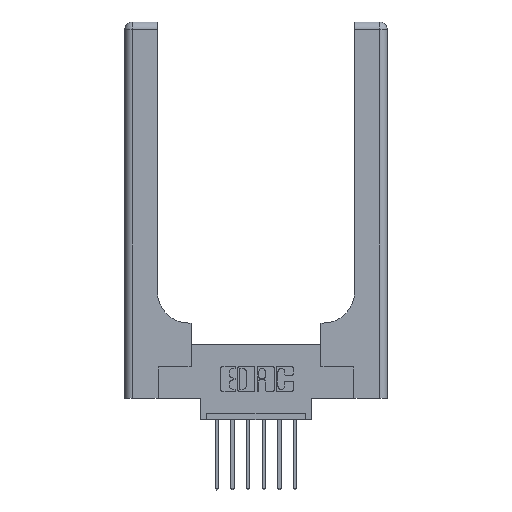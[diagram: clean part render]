
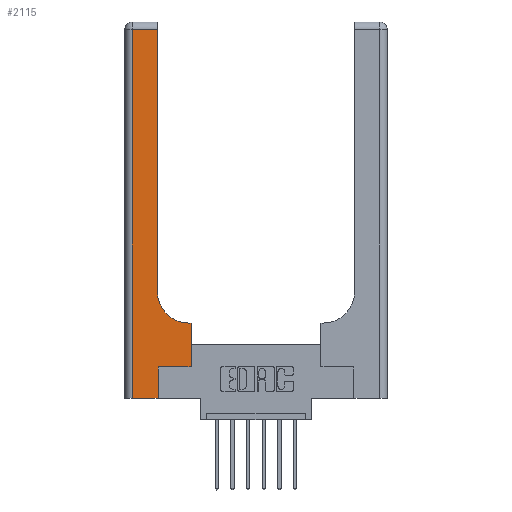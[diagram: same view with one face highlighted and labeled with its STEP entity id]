
A CAD part, top view. The second image highlights one B-rep face of the part: STEP entity #2115.
In plain terms, the highlighted planar face has unit normal (0, 0, 1).
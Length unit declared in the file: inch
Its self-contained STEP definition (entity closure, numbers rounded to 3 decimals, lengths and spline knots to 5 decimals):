
#15 = DIRECTION ( 'NONE',  ( 0., 1., 0. ) ) ;
#78 = CARTESIAN_POINT ( 'NONE',  ( 0., 2.94, 0.37 ) ) ;
#370 = CARTESIAN_POINT ( 'NONE',  ( 0.06, 3., 0.37 ) ) ;
#759 = ORIENTED_EDGE ( 'NONE', *, *, #9715, .T. ) ;
#881 = ORIENTED_EDGE ( 'NONE', *, *, #1555, .T. ) ;
#924 = CARTESIAN_POINT ( 'NONE',  ( 0.528, 0.25, 0.37 ) ) ;
#1103 = LINE ( 'NONE', #5512, #12631 ) ;
#1555 = EDGE_CURVE ( 'NONE', #10380, #11498, #8942, .T. ) ;
#1660 = CARTESIAN_POINT ( 'NONE',  ( 0., 3., 0.37 ) ) ;
#1914 = DIRECTION ( 'NONE',  ( -1., 0., 0. ) ) ;
#2111 = DIRECTION ( 'NONE',  ( 0., 1., 0. ) ) ;
#2115 = ADVANCED_FACE ( 'NONE', ( #11547 ), #7192, .F. ) ;
#2128 = ORIENTED_EDGE ( 'NONE', *, *, #14217, .T. ) ;
#2170 = ORIENTED_EDGE ( 'NONE', *, *, #10013, .T. ) ;
#2223 = LINE ( 'NONE', #6659, #11926 ) ;
#2560 = CARTESIAN_POINT ( 'NONE',  ( 0.26, 0.6, 0.37 ) ) ;
#2639 = VERTEX_POINT ( 'NONE', #3822 ) ;
#2807 = ORIENTED_EDGE ( 'NONE', *, *, #11978, .T. ) ;
#2943 = AXIS2_PLACEMENT_3D ( 'NONE', #1660, #6057, #10507 ) ;
#3070 = LINE ( 'NONE', #5226, #9410 ) ;
#3141 = CARTESIAN_POINT ( 'NONE',  ( 0., 0., 0.37 ) ) ;
#3278 = CARTESIAN_POINT ( 'NONE',  ( 0.06, 0., 0.37 ) ) ;
#3731 = ORIENTED_EDGE ( 'NONE', *, *, #12432, .T. ) ;
#3822 = CARTESIAN_POINT ( 'NONE',  ( 0.06, 2.94, 0.37 ) ) ;
#3961 = CARTESIAN_POINT ( 'NONE',  ( 0.26, 2.94, 0.37 ) ) ;
#4257 = CARTESIAN_POINT ( 'NONE',  ( 0.528, 0.25, 0.37 ) ) ;
#4281 = DIRECTION ( 'NONE',  ( 0., 1., 0. ) ) ;
#4335 = CARTESIAN_POINT ( 'NONE',  ( 0.51, 0.6, 0.37 ) ) ;
#4473 = LINE ( 'NONE', #4257, #9655 ) ;
#4679 = VERTEX_POINT ( 'NONE', #12156 ) ;
#4753 = EDGE_CURVE ( 'NONE', #10972, #11633, #3070, .T. ) ;
#5079 = VECTOR ( 'NONE', #7978, 39.37008 ) ;
#5094 = CARTESIAN_POINT ( 'NONE',  ( 0.265, 0., 0.37 ) ) ;
#5226 = CARTESIAN_POINT ( 'NONE',  ( 0.265, 0.25, 0.37 ) ) ;
#5512 = CARTESIAN_POINT ( 'NONE',  ( 0.26, 3., 0.37 ) ) ;
#5945 = LINE ( 'NONE', #370, #12302 ) ;
#6057 = DIRECTION ( 'NONE',  ( 0., 0., -1. ) ) ;
#6099 = CARTESIAN_POINT ( 'NONE',  ( 0.51, 0.85, 0.37 ) ) ;
#6241 = AXIS2_PLACEMENT_3D ( 'NONE', #6099, #12882, #13882 ) ;
#6659 = CARTESIAN_POINT ( 'NONE',  ( 0.265, 0., 0.37 ) ) ;
#7192 = PLANE ( 'NONE',  #2943 ) ;
#7372 = EDGE_CURVE ( 'NONE', #11462, #2639, #11117, .T. ) ;
#7378 = VERTEX_POINT ( 'NONE', #4335 ) ;
#7686 = ORIENTED_EDGE ( 'NONE', *, *, #7372, .T. ) ;
#7878 = EDGE_CURVE ( 'NONE', #4679, #7378, #11373, .T. ) ;
#7978 = DIRECTION ( 'NONE',  ( -1., 0., 0. ) ) ;
#8942 = LINE ( 'NONE', #3141, #12424 ) ;
#9410 = VECTOR ( 'NONE', #12783, 39.37008 ) ;
#9416 = ORIENTED_EDGE ( 'NONE', *, *, #4753, .T. ) ;
#9655 = VECTOR ( 'NONE', #2111, 39.37008 ) ;
#9715 = EDGE_CURVE ( 'NONE', #2639, #10380, #5945, .T. ) ;
#10013 = EDGE_CURVE ( 'NONE', #7378, #12301, #10428, .T. ) ;
#10380 = VERTEX_POINT ( 'NONE', #3278 ) ;
#10428 = CIRCLE ( 'NONE', #6241, 0.25 ) ;
#10507 = DIRECTION ( 'NONE',  ( -1., 0., 0. ) ) ;
#10972 = VERTEX_POINT ( 'NONE', #11123 ) ;
#11117 = LINE ( 'NONE', #78, #13640 ) ;
#11123 = CARTESIAN_POINT ( 'NONE',  ( 0.265, 0.25, 0.37 ) ) ;
#11373 = LINE ( 'NONE', #2560, #5079 ) ;
#11462 = VERTEX_POINT ( 'NONE', #3961 ) ;
#11497 = EDGE_LOOP ( 'NONE', ( #2807, #7686, #759, #881, #3731, #9416, #2128, #13932, #2170 ) ) ;
#11498 = VERTEX_POINT ( 'NONE', #5094 ) ;
#11547 = FACE_OUTER_BOUND ( 'NONE', #11497, .T. ) ;
#11633 = VERTEX_POINT ( 'NONE', #924 ) ;
#11926 = VECTOR ( 'NONE', #4281, 39.37008 ) ;
#11978 = EDGE_CURVE ( 'NONE', #12301, #11462, #1103, .T. ) ;
#12142 = DIRECTION ( 'NONE',  ( 1., 0., 0. ) ) ;
#12156 = CARTESIAN_POINT ( 'NONE',  ( 0.528, 0.6, 0.37 ) ) ;
#12301 = VERTEX_POINT ( 'NONE', #13981 ) ;
#12302 = VECTOR ( 'NONE', #12378, 39.37008 ) ;
#12378 = DIRECTION ( 'NONE',  ( 0., -1., 0. ) ) ;
#12424 = VECTOR ( 'NONE', #12142, 39.37008 ) ;
#12432 = EDGE_CURVE ( 'NONE', #11498, #10972, #2223, .T. ) ;
#12631 = VECTOR ( 'NONE', #15, 39.37008 ) ;
#12783 = DIRECTION ( 'NONE',  ( 1., 0., 0. ) ) ;
#12882 = DIRECTION ( 'NONE',  ( 0., 0., -1. ) ) ;
#13640 = VECTOR ( 'NONE', #1914, 39.37008 ) ;
#13882 = DIRECTION ( 'NONE',  ( 1., 0., 0. ) ) ;
#13932 = ORIENTED_EDGE ( 'NONE', *, *, #7878, .T. ) ;
#13981 = CARTESIAN_POINT ( 'NONE',  ( 0.26, 0.85, 0.37 ) ) ;
#14217 = EDGE_CURVE ( 'NONE', #11633, #4679, #4473, .T. ) ;
